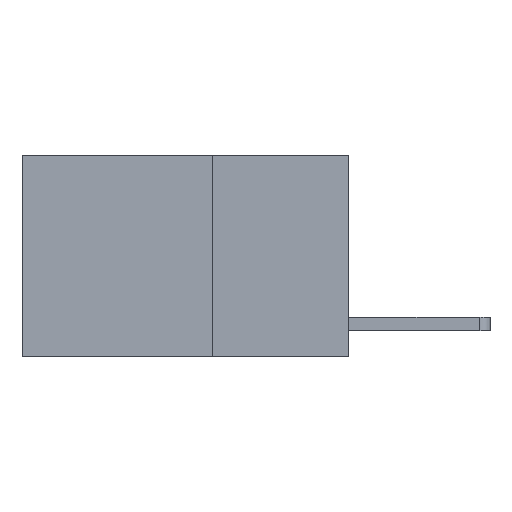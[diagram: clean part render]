
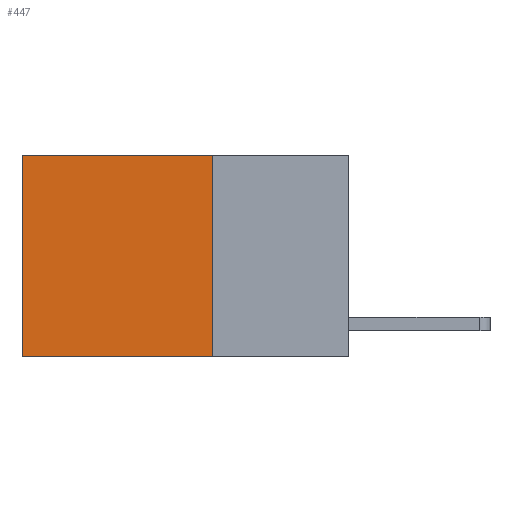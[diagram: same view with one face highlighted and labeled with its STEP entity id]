
A CAD part, left-side view. The second image highlights one B-rep face of the part: STEP entity #447.
In plain terms, the highlighted planar face has unit normal (-1, 0, 0).
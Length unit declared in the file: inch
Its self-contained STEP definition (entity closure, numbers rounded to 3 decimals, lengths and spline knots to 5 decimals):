
#447 = ADVANCED_FACE ( 'NONE', ( #4184 ), #8290, .F. ) ;
#689 = VERTEX_POINT ( 'NONE', #8335 ) ;
#842 = VECTOR ( 'NONE', #5057, 39.37008 ) ;
#2313 = VERTEX_POINT ( 'NONE', #9455 ) ;
#2525 = LINE ( 'NONE', #5539, #6367 ) ;
#2735 = VERTEX_POINT ( 'NONE', #6427 ) ;
#2816 = LINE ( 'NONE', #8623, #4405 ) ;
#2848 = DIRECTION ( 'NONE',  ( 0., 1., 0. ) ) ;
#3204 = CARTESIAN_POINT ( 'NONE',  ( 0.2625, 0.25, 0. ) ) ;
#3956 = EDGE_CURVE ( 'NONE', #2313, #689, #2525, .T. ) ;
#4075 = LINE ( 'NONE', #3204, #9964 ) ;
#4184 = FACE_OUTER_BOUND ( 'NONE', #9946, .T. ) ;
#4405 = VECTOR ( 'NONE', #8614, 39.37008 ) ;
#4500 = CARTESIAN_POINT ( 'NONE',  ( 0.2625, 0.25, -0.37 ) ) ;
#4538 = EDGE_CURVE ( 'NONE', #2313, #2735, #4075, .T. ) ;
#4757 = AXIS2_PLACEMENT_3D ( 'NONE', #6869, #8149, #8119 ) ;
#4917 = EDGE_CURVE ( 'NONE', #689, #6916, #7051, .T. ) ;
#5057 = DIRECTION ( 'NONE',  ( 0., 1., 0. ) ) ;
#5539 = CARTESIAN_POINT ( 'NONE',  ( 0.2625, 0.25, 0. ) ) ;
#5907 = ORIENTED_EDGE ( 'NONE', *, *, #7958, .T. ) ;
#5924 = ORIENTED_EDGE ( 'NONE', *, *, #4917, .F. ) ;
#5949 = ORIENTED_EDGE ( 'NONE', *, *, #3956, .F. ) ;
#6116 = ORIENTED_EDGE ( 'NONE', *, *, #4538, .T. ) ;
#6367 = VECTOR ( 'NONE', #9889, 39.37008 ) ;
#6427 = CARTESIAN_POINT ( 'NONE',  ( 0.2625, 0.6, 0. ) ) ;
#6869 = CARTESIAN_POINT ( 'NONE',  ( 0.2625, 0.25, 0. ) ) ;
#6916 = VERTEX_POINT ( 'NONE', #7945 ) ;
#7051 = LINE ( 'NONE', #4500, #842 ) ;
#7945 = CARTESIAN_POINT ( 'NONE',  ( 0.2625, 0.6, -0.37 ) ) ;
#7958 = EDGE_CURVE ( 'NONE', #2735, #6916, #2816, .T. ) ;
#8119 = DIRECTION ( 'NONE',  ( 0., 0., -1. ) ) ;
#8149 = DIRECTION ( 'NONE',  ( 1., 0., 0. ) ) ;
#8290 = PLANE ( 'NONE',  #4757 ) ;
#8335 = CARTESIAN_POINT ( 'NONE',  ( 0.2625, 0.25, -0.37 ) ) ;
#8614 = DIRECTION ( 'NONE',  ( 0., 0., -1. ) ) ;
#8623 = CARTESIAN_POINT ( 'NONE',  ( 0.2625, 0.6, 0. ) ) ;
#9455 = CARTESIAN_POINT ( 'NONE',  ( 0.2625, 0.25, 0. ) ) ;
#9889 = DIRECTION ( 'NONE',  ( 0., 0., -1. ) ) ;
#9946 = EDGE_LOOP ( 'NONE', ( #5907, #5924, #5949, #6116 ) ) ;
#9964 = VECTOR ( 'NONE', #2848, 39.37008 ) ;
